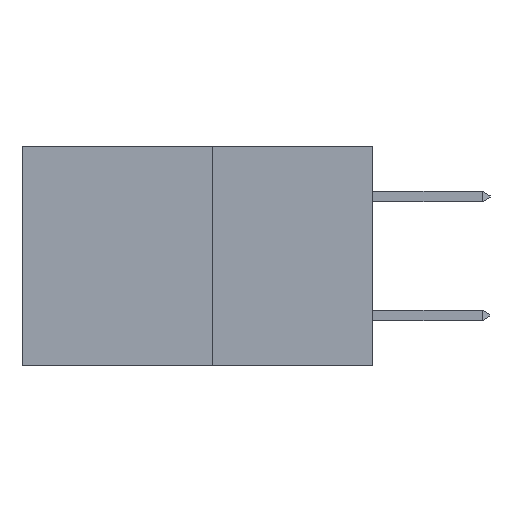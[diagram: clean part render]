
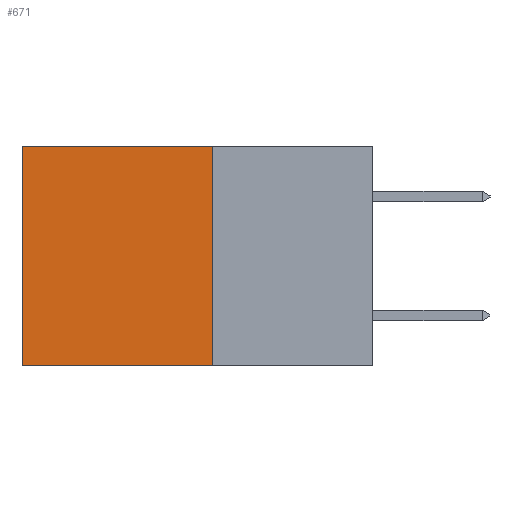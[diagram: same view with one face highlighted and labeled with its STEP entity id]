
A CAD part, left-side view. The second image highlights one B-rep face of the part: STEP entity #671.
In plain terms, the highlighted planar face has unit normal (-1, 0, 0).
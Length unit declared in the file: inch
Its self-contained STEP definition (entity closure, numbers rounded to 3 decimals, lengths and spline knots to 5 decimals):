
#671 = ADVANCED_FACE ( 'NONE', ( #6780 ), #11597, .F. ) ;
#1122 = EDGE_CURVE ( 'NONE', #12689, #9883, #7424, .T. ) ;
#1242 = AXIS2_PLACEMENT_3D ( 'NONE', #7684, #13420, #8228 ) ;
#2349 = EDGE_CURVE ( 'NONE', #11487, #12689, #5299, .T. ) ;
#2625 = ORIENTED_EDGE ( 'NONE', *, *, #2747, .F. ) ;
#2747 = EDGE_CURVE ( 'NONE', #13517, #9883, #5289, .T. ) ;
#2805 = CARTESIAN_POINT ( 'NONE',  ( 0.277, 0.59, -0.37 ) ) ;
#4025 = CARTESIAN_POINT ( 'NONE',  ( 0.277, 0.27, 0. ) ) ;
#4063 = DIRECTION ( 'NONE',  ( 0., 0., -1. ) ) ;
#4126 = DIRECTION ( 'NONE',  ( 0., 0., -1. ) ) ;
#4917 = VECTOR ( 'NONE', #4126, 39.37008 ) ;
#5240 = LINE ( 'NONE', #10871, #4917 ) ;
#5289 = LINE ( 'NONE', #7920, #10612 ) ;
#5299 = LINE ( 'NONE', #4025, #7721 ) ;
#5364 = EDGE_CURVE ( 'NONE', #11487, #13517, #5240, .T. ) ;
#5535 = DIRECTION ( 'NONE',  ( 0., 1., 0. ) ) ;
#6238 = ORIENTED_EDGE ( 'NONE', *, *, #5364, .F. ) ;
#6780 = FACE_OUTER_BOUND ( 'NONE', #12178, .T. ) ;
#7416 = CARTESIAN_POINT ( 'NONE',  ( 0.277, 0.27, 0. ) ) ;
#7424 = LINE ( 'NONE', #2805, #13123 ) ;
#7684 = CARTESIAN_POINT ( 'NONE',  ( 0.277, 0.27, -0.37 ) ) ;
#7721 = VECTOR ( 'NONE', #5535, 39.37008 ) ;
#7900 = ORIENTED_EDGE ( 'NONE', *, *, #1122, .T. ) ;
#7920 = CARTESIAN_POINT ( 'NONE',  ( 0.277, 0.27, -0.37 ) ) ;
#8228 = DIRECTION ( 'NONE',  ( 0., 0., -1. ) ) ;
#8536 = DIRECTION ( 'NONE',  ( 0., 1., 0. ) ) ;
#8669 = CARTESIAN_POINT ( 'NONE',  ( 0.277, 0.59, -0.37 ) ) ;
#9441 = CARTESIAN_POINT ( 'NONE',  ( 0.277, 0.59, 0. ) ) ;
#9883 = VERTEX_POINT ( 'NONE', #8669 ) ;
#10612 = VECTOR ( 'NONE', #8536, 39.37008 ) ;
#10871 = CARTESIAN_POINT ( 'NONE',  ( 0.277, 0.27, -0.37 ) ) ;
#11382 = ORIENTED_EDGE ( 'NONE', *, *, #2349, .T. ) ;
#11487 = VERTEX_POINT ( 'NONE', #7416 ) ;
#11597 = PLANE ( 'NONE',  #1242 ) ;
#11717 = CARTESIAN_POINT ( 'NONE',  ( 0.277, 0.27, -0.37 ) ) ;
#12178 = EDGE_LOOP ( 'NONE', ( #7900, #2625, #6238, #11382 ) ) ;
#12689 = VERTEX_POINT ( 'NONE', #9441 ) ;
#13123 = VECTOR ( 'NONE', #4063, 39.37008 ) ;
#13420 = DIRECTION ( 'NONE',  ( 1., 0., 0. ) ) ;
#13517 = VERTEX_POINT ( 'NONE', #11717 ) ;
